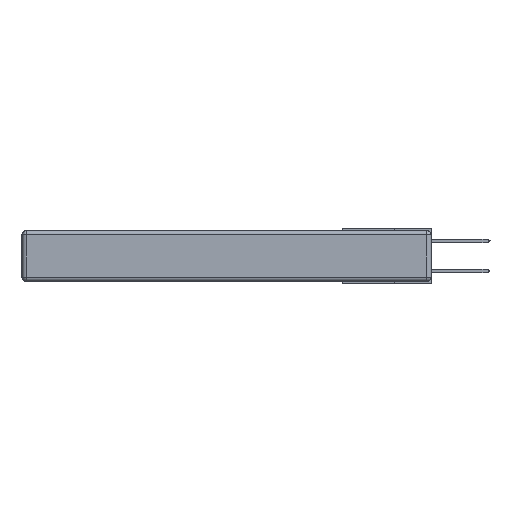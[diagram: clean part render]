
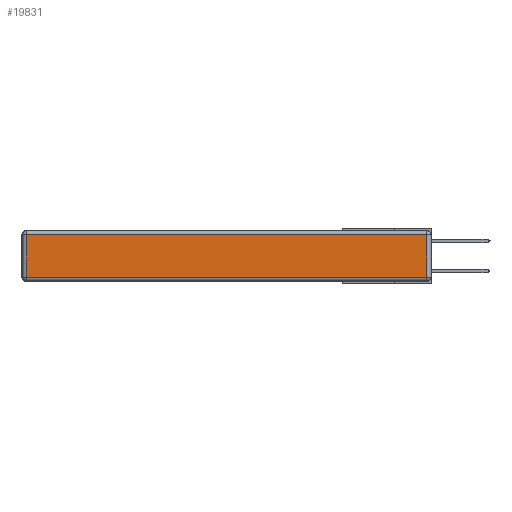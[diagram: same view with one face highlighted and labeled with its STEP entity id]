
A CAD part, left-side view. The second image highlights one B-rep face of the part: STEP entity #19831.
In plain terms, the highlighted planar face has unit normal (-1, 0, 0).
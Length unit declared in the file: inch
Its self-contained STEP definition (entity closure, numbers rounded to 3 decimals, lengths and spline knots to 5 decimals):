
#1516 = ORIENTED_EDGE ( 'NONE', *, *, #8288, .T. ) ;
#1618 = CARTESIAN_POINT ( 'NONE',  ( 0., 2.72, -0.313 ) ) ;
#1823 = LINE ( 'NONE', #15961, #18435 ) ;
#2283 = FACE_OUTER_BOUND ( 'NONE', #22776, .T. ) ;
#2500 = CARTESIAN_POINT ( 'NONE',  ( 0., 2.72, -0.343 ) ) ;
#2667 = ORIENTED_EDGE ( 'NONE', *, *, #19254, .T. ) ;
#2833 = VERTEX_POINT ( 'NONE', #1618 ) ;
#3421 = CARTESIAN_POINT ( 'NONE',  ( 0., 0.03, -0.313 ) ) ;
#3509 = DIRECTION ( 'NONE',  ( -1., 0., 0. ) ) ;
#3678 = VECTOR ( 'NONE', #12871, 39.37008 ) ;
#3945 = ORIENTED_EDGE ( 'NONE', *, *, #12017, .T. ) ;
#4070 = VECTOR ( 'NONE', #11760, 39.37008 ) ;
#4892 = LINE ( 'NONE', #2500, #4070 ) ;
#6509 = LINE ( 'NONE', #14864, #3678 ) ;
#6862 = CARTESIAN_POINT ( 'NONE',  ( 0., 2.72, -0.03 ) ) ;
#8288 = EDGE_CURVE ( 'NONE', #18885, #2833, #4892, .T. ) ;
#10825 = DIRECTION ( 'NONE',  ( 0., 0., 1. ) ) ;
#11760 = DIRECTION ( 'NONE',  ( 0., 0., -1. ) ) ;
#12017 = EDGE_CURVE ( 'NONE', #21522, #15197, #1823, .T. ) ;
#12467 = CARTESIAN_POINT ( 'NONE',  ( 0., 0.03, -0.03 ) ) ;
#12871 = DIRECTION ( 'NONE',  ( 0., -1., 0. ) ) ;
#12979 = AXIS2_PLACEMENT_3D ( 'NONE', #20146, #3509, #10825 ) ;
#13282 = DIRECTION ( 'NONE',  ( 0., 1., 0. ) ) ;
#14864 = CARTESIAN_POINT ( 'NONE',  ( 0., 0., -0.313 ) ) ;
#15197 = VERTEX_POINT ( 'NONE', #12467 ) ;
#15465 = VECTOR ( 'NONE', #13282, 39.37008 ) ;
#15483 = EDGE_CURVE ( 'NONE', #2833, #21522, #6509, .T. ) ;
#15961 = CARTESIAN_POINT ( 'NONE',  ( 0., 0.03, -0.343 ) ) ;
#17124 = CARTESIAN_POINT ( 'NONE',  ( 0., 2.75, -0.03 ) ) ;
#18435 = VECTOR ( 'NONE', #19666, 39.37008 ) ;
#18885 = VERTEX_POINT ( 'NONE', #6862 ) ;
#19254 = EDGE_CURVE ( 'NONE', #15197, #18885, #20357, .T. ) ;
#19666 = DIRECTION ( 'NONE',  ( 0., 0., 1. ) ) ;
#19831 = ADVANCED_FACE ( 'NONE', ( #2283 ), #23670, .T. ) ;
#20146 = CARTESIAN_POINT ( 'NONE',  ( 0., 0., -0.343 ) ) ;
#20357 = LINE ( 'NONE', #17124, #15465 ) ;
#20405 = ORIENTED_EDGE ( 'NONE', *, *, #15483, .T. ) ;
#21522 = VERTEX_POINT ( 'NONE', #3421 ) ;
#22776 = EDGE_LOOP ( 'NONE', ( #20405, #3945, #2667, #1516 ) ) ;
#23670 = PLANE ( 'NONE',  #12979 ) ;
